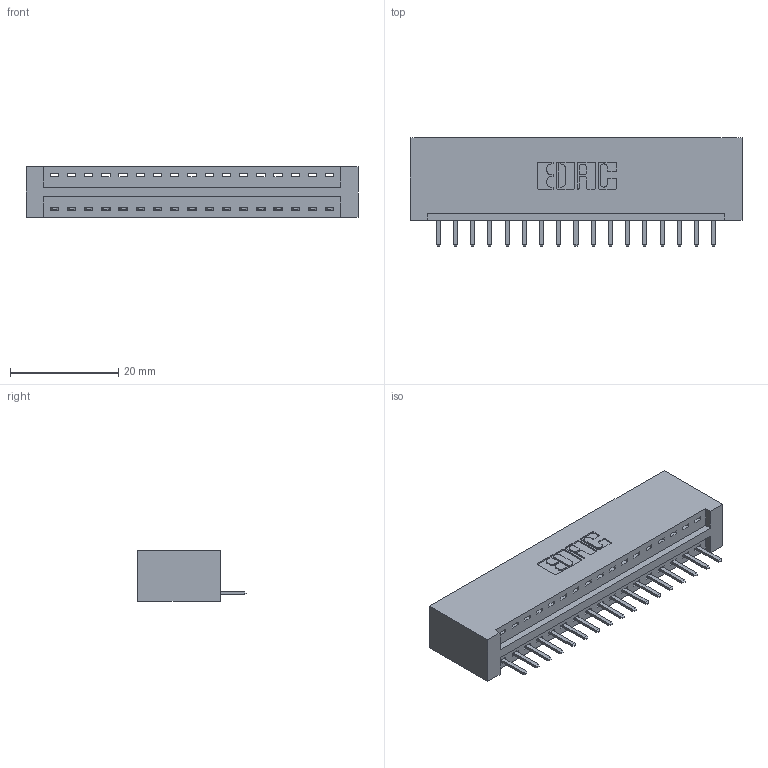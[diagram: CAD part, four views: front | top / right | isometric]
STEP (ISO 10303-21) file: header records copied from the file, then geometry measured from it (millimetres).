
FILE_DESCRIPTION (( 'STEP AP203' ), '1' );
FILE_NAME ('346-017-520-101.STEP', '2022-05-05T11:34:06', ( '' ), ( '' ), 'SwSTEP 2.0', 'SolidWorks 2020', '' );
FILE_SCHEMA (( 'CONFIG_CONTROL_DESIGN' ));
Length unit declared in the file: inch
Products named in the file (3): 346-017-520-101; 345-292-001_345-293-120; 346 Part_No Mounting Lugs
Assembly tree (18 placements, depth 2):
  346-017-520-101
    346 Part_No Mounting Lugs
    345-292-001_345-293-120  x17
Bounding box: 61.21 x 20.02 x 9.4 mm (x, y, z)
Volume: 6187.8 mm3; surface area: 7376 mm2
Topology: 18 solids, 18 shells, 1168 faces, 3433 edges, 2242 vertices
Faces by surface type: plane 786, cylinder 382
Entity records: 13753 total; most frequent: CARTESIAN_POINT 2383, ORIENTED_EDGE 2322, DIRECTION 2115, EDGE_CURVE 1161, LINE 965, VECTOR 965, VERTEX_POINT 770, AXIS2_PLACEMENT_3D 575
